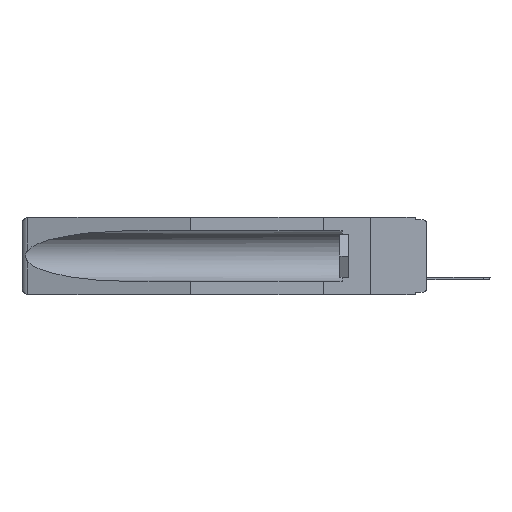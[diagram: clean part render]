
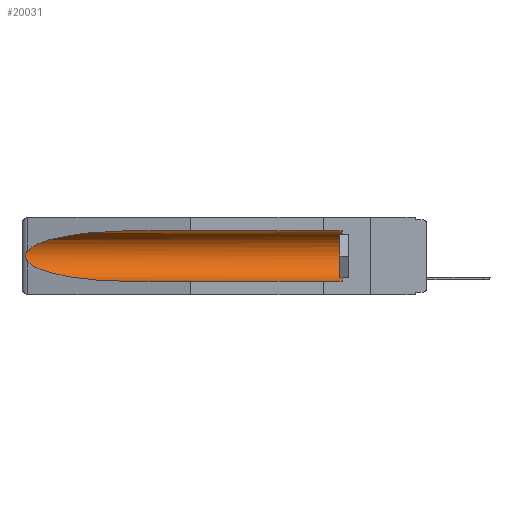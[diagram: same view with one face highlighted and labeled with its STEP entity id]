
A CAD part, left-side view. The second image highlights one B-rep face of the part: STEP entity #20031.
In plain terms, the highlighted cylindrical face has radius 2.857 mm (diameter 5.715 mm), a partial arc.
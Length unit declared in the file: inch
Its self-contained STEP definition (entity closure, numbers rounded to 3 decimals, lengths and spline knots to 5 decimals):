
#551 = VERTEX_POINT ( 'NONE', #7883 ) ;
#801 = CARTESIAN_POINT ( 'NONE',  ( 0.2673, 1.53269, -0.17917 ) ) ;
#913 = CARTESIAN_POINT ( 'NONE',  ( 0.2675, 1.53308, -0.16763 ) ) ;
#2845 = CARTESIAN_POINT ( 'NONE',  ( 0.26597, 1.5296, -0.19026 ) ) ;
#3090 = CARTESIAN_POINT ( 'NONE',  ( 0.21114, 1.30732, -0.284 ) ) ;
#3623 = AXIS2_PLACEMENT_3D ( 'NONE', #8946, #18329, #12687 ) ;
#3754 =( BOUNDED_CURVE ( )  B_SPLINE_CURVE ( 3, ( #14134, #8252, #3090, #13775 ),
 .UNSPECIFIED., .F., .T. ) 
 B_SPLINE_CURVE_WITH_KNOTS ( ( 4, 4 ),
 ( 0.1948, 1.5708 ),
 .UNSPECIFIED. ) 
 CURVE ( )  GEOMETRIC_REPRESENTATION_ITEM ( )  RATIONAL_B_SPLINE_CURVE ( ( 1., 0.848, 0.848, 1. ) ) 
 REPRESENTATION_ITEM ( '' )  );
#3783 = ORIENTED_EDGE ( 'NONE', *, *, #6721, .T. ) ;
#3851 = LINE ( 'NONE', #18740, #5169 ) ;
#4067 = AXIS2_PLACEMENT_3D ( 'NONE', #5805, #20806, #17092 ) ;
#4704 = ORIENTED_EDGE ( 'NONE', *, *, #9263, .T. ) ;
#5169 = VECTOR ( 'NONE', #9480, 39.37008 ) ;
#5410 = CARTESIAN_POINT ( 'NONE',  ( 0.21114, 1.30732, -0.059 ) ) ;
#5805 = CARTESIAN_POINT ( 'NONE',  ( 0.155, -0.30754, -0.1715 ) ) ;
#6036 = CYLINDRICAL_SURFACE ( 'NONE', #4067, 0.1125 ) ;
#6451 = CARTESIAN_POINT ( 'NONE',  ( 0.26537, 1.52718, -0.19328 ) ) ;
#6471 = CARTESIAN_POINT ( 'NONE',  ( 0.155, 0.126, -0.284 ) ) ;
#6677 = CARTESIAN_POINT ( 'NONE',  ( 0.2673, 1.5327, -0.16383 ) ) ;
#6721 = EDGE_CURVE ( 'NONE', #22116, #551, #13815, .T. ) ;
#7192 = EDGE_LOOP ( 'NONE', ( #4704, #3783, #14298, #10257, #14694, #16447 ) ) ;
#7883 = CARTESIAN_POINT ( 'NONE',  ( 0.26537, 1.52718, -0.19328 ) ) ;
#8035 = EDGE_CURVE ( 'NONE', #551, #21991, #3754, .T. ) ;
#8131 = CARTESIAN_POINT ( 'NONE',  ( 0.155, -0.30754, -0.284 ) ) ;
#8252 = CARTESIAN_POINT ( 'NONE',  ( 0.25451, 1.48313, -0.24835 ) ) ;
#8946 = CARTESIAN_POINT ( 'NONE',  ( 0.155, 0.126, -0.1715 ) ) ;
#9263 = EDGE_CURVE ( 'NONE', #19051, #22116, #19396, .T. ) ;
#9480 = DIRECTION ( 'NONE',  ( 0., 1., 0. ) ) ;
#10161 = LINE ( 'NONE', #8131, #10713 ) ;
#10216 = EDGE_CURVE ( 'NONE', #13375, #17304, #13972, .T. ) ;
#10257 = ORIENTED_EDGE ( 'NONE', *, *, #16441, .F. ) ;
#10713 = VECTOR ( 'NONE', #22560, 39.37008 ) ;
#11046 = CARTESIAN_POINT ( 'NONE',  ( 0.155, 1.07973, -0.059 ) ) ;
#12687 = DIRECTION ( 'NONE',  ( 0., 0., 1. ) ) ;
#13375 = VERTEX_POINT ( 'NONE', #6471 ) ;
#13770 = CARTESIAN_POINT ( 'NONE',  ( 0.26537, 1.52718, -0.14972 ) ) ;
#13775 = CARTESIAN_POINT ( 'NONE',  ( 0.155, 1.07973, -0.284 ) ) ;
#13815 = B_SPLINE_CURVE_WITH_KNOTS ( 'NONE', 3,
 ( #13770, #20981, #17615, #6677, #913, #19302, #801, #19188, #2845, #6451 ),
 .UNSPECIFIED., .F., .F.,
 ( 4, 2, 2, 2, 4 ),
 ( 0., 0.00029, 0.00058, 0.00087, 0.00117 ),
 .UNSPECIFIED. ) ;
#13972 = CIRCLE ( 'NONE', #3623, 0.1125 ) ;
#14134 = CARTESIAN_POINT ( 'NONE',  ( 0.26537, 1.52718, -0.19328 ) ) ;
#14298 = ORIENTED_EDGE ( 'NONE', *, *, #8035, .T. ) ;
#14694 = ORIENTED_EDGE ( 'NONE', *, *, #10216, .T. ) ;
#15130 = CARTESIAN_POINT ( 'NONE',  ( 0.155, 1.07973, -0.059 ) ) ;
#15399 = CARTESIAN_POINT ( 'NONE',  ( 0.155, 0.126, -0.059 ) ) ;
#16213 = CARTESIAN_POINT ( 'NONE',  ( 0.26537, 1.52718, -0.14972 ) ) ;
#16441 = EDGE_CURVE ( 'NONE', #13375, #21991, #10161, .T. ) ;
#16447 = ORIENTED_EDGE ( 'NONE', *, *, #19100, .T. ) ;
#17092 = DIRECTION ( 'NONE',  ( 0., 0., 1. ) ) ;
#17304 = VERTEX_POINT ( 'NONE', #15399 ) ;
#17615 = CARTESIAN_POINT ( 'NONE',  ( 0.26654, 1.53092, -0.15636 ) ) ;
#18329 = DIRECTION ( 'NONE',  ( 0., -1., 0. ) ) ;
#18385 = CARTESIAN_POINT ( 'NONE',  ( 0.25451, 1.48313, -0.09465 ) ) ;
#18740 = CARTESIAN_POINT ( 'NONE',  ( 0.155, -0.30754, -0.059 ) ) ;
#19051 = VERTEX_POINT ( 'NONE', #15130 ) ;
#19100 = EDGE_CURVE ( 'NONE', #17304, #19051, #3851, .T. ) ;
#19188 = CARTESIAN_POINT ( 'NONE',  ( 0.26655, 1.53094, -0.18657 ) ) ;
#19302 = CARTESIAN_POINT ( 'NONE',  ( 0.2675, 1.53308, -0.17534 ) ) ;
#19396 =( BOUNDED_CURVE ( )  B_SPLINE_CURVE ( 3, ( #11046, #5410, #18385, #16213 ),
 .UNSPECIFIED., .F., .F. ) 
 B_SPLINE_CURVE_WITH_KNOTS ( ( 4, 4 ),
 ( 4.71239, 6.08839 ),
 .UNSPECIFIED. ) 
 CURVE ( )  GEOMETRIC_REPRESENTATION_ITEM ( )  RATIONAL_B_SPLINE_CURVE ( ( 1., 0.848, 0.848, 1. ) ) 
 REPRESENTATION_ITEM ( '' )  );
#20031 = ADVANCED_FACE ( 'NONE', ( #22256 ), #6036, .F. ) ;
#20806 = DIRECTION ( 'NONE',  ( 0., 1., 0. ) ) ;
#20981 = CARTESIAN_POINT ( 'NONE',  ( 0.26597, 1.52961, -0.15275 ) ) ;
#21348 = CARTESIAN_POINT ( 'NONE',  ( 0.155, 1.07973, -0.284 ) ) ;
#21991 = VERTEX_POINT ( 'NONE', #21348 ) ;
#22116 = VERTEX_POINT ( 'NONE', #22175 ) ;
#22175 = CARTESIAN_POINT ( 'NONE',  ( 0.26537, 1.52718, -0.14972 ) ) ;
#22256 = FACE_OUTER_BOUND ( 'NONE', #7192, .T. ) ;
#22560 = DIRECTION ( 'NONE',  ( 0., 1., 0. ) ) ;
